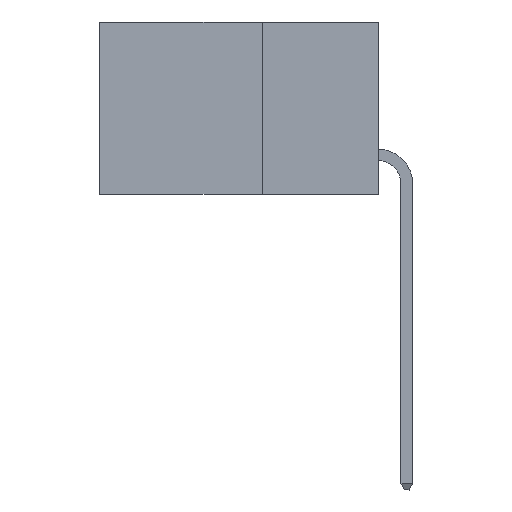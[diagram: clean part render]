
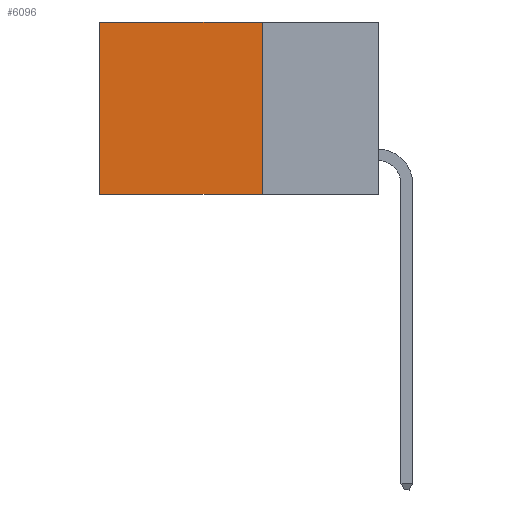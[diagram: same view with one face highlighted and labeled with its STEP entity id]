
A CAD part, left-side view. The second image highlights one B-rep face of the part: STEP entity #6096.
In plain terms, the highlighted planar face has unit normal (-1, 0, 0).
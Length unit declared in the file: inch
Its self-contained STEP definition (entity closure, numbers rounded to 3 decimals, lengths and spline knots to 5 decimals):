
#202 = LINE ( 'NONE', #5952, #7119 ) ;
#862 = CARTESIAN_POINT ( 'NONE',  ( 0.2615, 0.25, -0.37 ) ) ;
#1804 = PLANE ( 'NONE',  #4453 ) ;
#2331 = CARTESIAN_POINT ( 'NONE',  ( 0.2615, 0.6, -0.37 ) ) ;
#2940 = VECTOR ( 'NONE', #9508, 39.37008 ) ;
#3306 = EDGE_LOOP ( 'NONE', ( #16271, #8198, #6925, #11398 ) ) ;
#3754 = LINE ( 'NONE', #18069, #6906 ) ;
#3788 = DIRECTION ( 'NONE',  ( 0., 0., -1. ) ) ;
#4060 = DIRECTION ( 'NONE',  ( 1., 0., 0. ) ) ;
#4453 = AXIS2_PLACEMENT_3D ( 'NONE', #12216, #4060, #3788 ) ;
#4554 = DIRECTION ( 'NONE',  ( 0., 1., 0. ) ) ;
#4661 = VECTOR ( 'NONE', #15981, 39.37008 ) ;
#5237 = DIRECTION ( 'NONE',  ( 0., 0., -1. ) ) ;
#5413 = EDGE_CURVE ( 'NONE', #17358, #11160, #202, .T. ) ;
#5485 = EDGE_CURVE ( 'NONE', #9938, #16064, #7727, .T. ) ;
#5952 = CARTESIAN_POINT ( 'NONE',  ( 0.2615, 0.25, 0. ) ) ;
#6096 = ADVANCED_FACE ( 'NONE', ( #8948 ), #1804, .F. ) ;
#6906 = VECTOR ( 'NONE', #5237, 39.37008 ) ;
#6925 = ORIENTED_EDGE ( 'NONE', *, *, #9859, .F. ) ;
#7119 = VECTOR ( 'NONE', #4554, 39.37008 ) ;
#7727 = LINE ( 'NONE', #862, #2940 ) ;
#8198 = ORIENTED_EDGE ( 'NONE', *, *, #5485, .F. ) ;
#8948 = FACE_OUTER_BOUND ( 'NONE', #3306, .T. ) ;
#9508 = DIRECTION ( 'NONE',  ( 0., 1., 0. ) ) ;
#9859 = EDGE_CURVE ( 'NONE', #17358, #9938, #3754, .T. ) ;
#9938 = VERTEX_POINT ( 'NONE', #15962 ) ;
#11160 = VERTEX_POINT ( 'NONE', #16546 ) ;
#11398 = ORIENTED_EDGE ( 'NONE', *, *, #5413, .T. ) ;
#12216 = CARTESIAN_POINT ( 'NONE',  ( 0.2615, 0.25, -0.37 ) ) ;
#12363 = CARTESIAN_POINT ( 'NONE',  ( 0.2615, 0.25, 0. ) ) ;
#13871 = EDGE_CURVE ( 'NONE', #11160, #16064, #17746, .T. ) ;
#15962 = CARTESIAN_POINT ( 'NONE',  ( 0.2615, 0.25, -0.37 ) ) ;
#15981 = DIRECTION ( 'NONE',  ( 0., 0., -1. ) ) ;
#16064 = VERTEX_POINT ( 'NONE', #2331 ) ;
#16254 = CARTESIAN_POINT ( 'NONE',  ( 0.2615, 0.6, -0.37 ) ) ;
#16271 = ORIENTED_EDGE ( 'NONE', *, *, #13871, .T. ) ;
#16546 = CARTESIAN_POINT ( 'NONE',  ( 0.2615, 0.6, 0. ) ) ;
#17358 = VERTEX_POINT ( 'NONE', #12363 ) ;
#17746 = LINE ( 'NONE', #16254, #4661 ) ;
#18069 = CARTESIAN_POINT ( 'NONE',  ( 0.2615, 0.25, -0.37 ) ) ;
